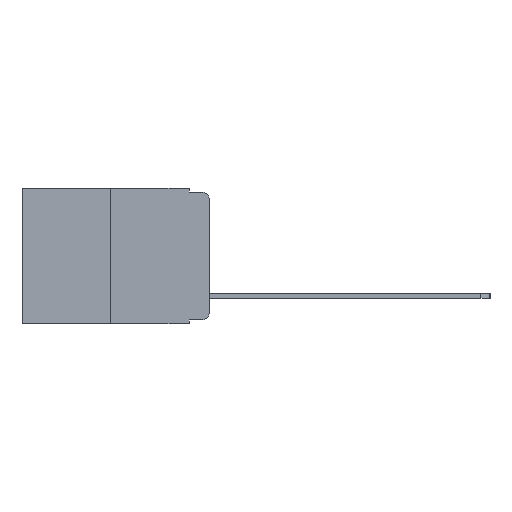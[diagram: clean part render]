
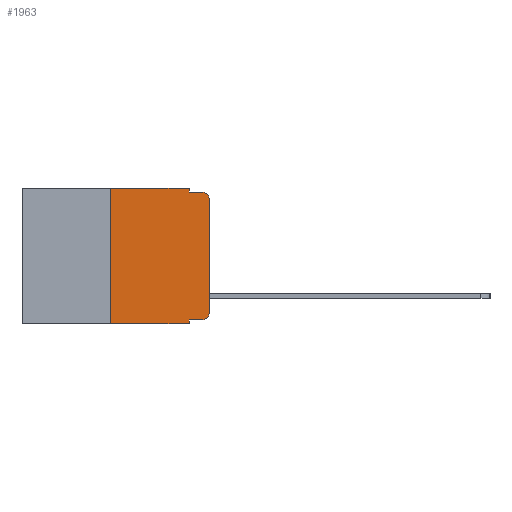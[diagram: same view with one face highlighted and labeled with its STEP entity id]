
A CAD part, left-side view. The second image highlights one B-rep face of the part: STEP entity #1963.
In plain terms, the highlighted planar face has unit normal (-1, 0, 0).
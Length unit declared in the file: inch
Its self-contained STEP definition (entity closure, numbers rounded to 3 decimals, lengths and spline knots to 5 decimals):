
#186 = DIRECTION ( 'NONE',  ( 0., 0., 1. ) ) ;
#354 = CARTESIAN_POINT ( 'NONE',  ( 0., 0.25, 0. ) ) ;
#454 = CARTESIAN_POINT ( 'NONE',  ( 0., 0.051, 0. ) ) ;
#1043 = CARTESIAN_POINT ( 'NONE',  ( 0., 0.02, -0.313 ) ) ;
#1963 = ADVANCED_FACE ( 'NONE', ( #18475 ), #14191, .F. ) ;
#1985 = ORIENTED_EDGE ( 'NONE', *, *, #7393, .T. ) ;
#2136 = DIRECTION ( 'NONE',  ( 1., 0., 0. ) ) ;
#2278 = DIRECTION ( 'NONE',  ( 0., 0., 1. ) ) ;
#2661 = AXIS2_PLACEMENT_3D ( 'NONE', #5911, #2136, #14071 ) ;
#2663 = CARTESIAN_POINT ( 'NONE',  ( 0., 0.02, -0.333 ) ) ;
#2836 = VERTEX_POINT ( 'NONE', #2663 ) ;
#3315 = AXIS2_PLACEMENT_3D ( 'NONE', #15085, #21780, #11551 ) ;
#3350 = EDGE_CURVE ( 'NONE', #8012, #16950, #9375, .T. ) ;
#3798 = EDGE_CURVE ( 'NONE', #2836, #16119, #5721, .T. ) ;
#3980 = EDGE_CURVE ( 'NONE', #20846, #5091, #10677, .T. ) ;
#4271 = DIRECTION ( 'NONE',  ( 0., 0., -1. ) ) ;
#5091 = VERTEX_POINT ( 'NONE', #18103 ) ;
#5386 = ORIENTED_EDGE ( 'NONE', *, *, #3980, .T. ) ;
#5599 = VECTOR ( 'NONE', #2278, 39.37008 ) ;
#5721 = CIRCLE ( 'NONE', #10090, 0.02 ) ;
#5911 = CARTESIAN_POINT ( 'NONE',  ( 0., 0.473, 0. ) ) ;
#6305 = LINE ( 'NONE', #6767, #14699 ) ;
#6406 = CARTESIAN_POINT ( 'NONE',  ( 0., 0.051, -0.01 ) ) ;
#6421 = ORIENTED_EDGE ( 'NONE', *, *, #3350, .T. ) ;
#6767 = CARTESIAN_POINT ( 'NONE',  ( 0., 0.051, -0.333 ) ) ;
#6988 = EDGE_CURVE ( 'NONE', #16119, #8012, #14178, .T. ) ;
#7312 = ORIENTED_EDGE ( 'NONE', *, *, #13431, .F. ) ;
#7393 = EDGE_CURVE ( 'NONE', #10416, #2836, #6305, .T. ) ;
#7529 = CARTESIAN_POINT ( 'NONE',  ( 0., 0., 0. ) ) ;
#7538 = ORIENTED_EDGE ( 'NONE', *, *, #14615, .F. ) ;
#7574 = EDGE_LOOP ( 'NONE', ( #19333, #6421, #14549, #7538, #20152, #7312, #5386, #12990, #1985, #10213 ) ) ;
#8012 = VERTEX_POINT ( 'NONE', #19024 ) ;
#8112 = LINE ( 'NONE', #11455, #21451 ) ;
#8447 = DIRECTION ( 'NONE',  ( 0., -1., 0. ) ) ;
#9168 = LINE ( 'NONE', #14069, #21903 ) ;
#9375 = CIRCLE ( 'NONE', #3315, 0.02 ) ;
#9409 = VECTOR ( 'NONE', #186, 39.37008 ) ;
#9461 = LINE ( 'NONE', #454, #18765 ) ;
#9604 = DIRECTION ( 'NONE',  ( 0., 0., -1. ) ) ;
#9836 = EDGE_CURVE ( 'NONE', #10416, #5091, #8112, .T. ) ;
#10090 = AXIS2_PLACEMENT_3D ( 'NONE', #1043, #11986, #22185 ) ;
#10213 = ORIENTED_EDGE ( 'NONE', *, *, #3798, .T. ) ;
#10416 = VERTEX_POINT ( 'NONE', #19391 ) ;
#10677 = LINE ( 'NONE', #14719, #13725 ) ;
#11455 = CARTESIAN_POINT ( 'NONE',  ( 0., 0.051, 0. ) ) ;
#11551 = DIRECTION ( 'NONE',  ( 0., 0., -1. ) ) ;
#11986 = DIRECTION ( 'NONE',  ( -1., 0., 0. ) ) ;
#12121 = CARTESIAN_POINT ( 'NONE',  ( 0., 0., -0.313 ) ) ;
#12556 = CARTESIAN_POINT ( 'NONE',  ( 0., 0.25, -0.343 ) ) ;
#12990 = ORIENTED_EDGE ( 'NONE', *, *, #9836, .F. ) ;
#13255 = VERTEX_POINT ( 'NONE', #22770 ) ;
#13431 = EDGE_CURVE ( 'NONE', #20846, #14871, #15656, .T. ) ;
#13725 = VECTOR ( 'NONE', #8447, 39.37008 ) ;
#14069 = CARTESIAN_POINT ( 'NONE',  ( 0., 0.051, -0.01 ) ) ;
#14071 = DIRECTION ( 'NONE',  ( 0., 0., -1. ) ) ;
#14178 = LINE ( 'NONE', #7529, #9409 ) ;
#14191 = PLANE ( 'NONE',  #2661 ) ;
#14229 = VECTOR ( 'NONE', #20067, 39.37008 ) ;
#14549 = ORIENTED_EDGE ( 'NONE', *, *, #18069, .F. ) ;
#14615 = EDGE_CURVE ( 'NONE', #13255, #19472, #9461, .T. ) ;
#14699 = VECTOR ( 'NONE', #20732, 39.37008 ) ;
#14719 = CARTESIAN_POINT ( 'NONE',  ( 0., 0.473, -0.343 ) ) ;
#14871 = VERTEX_POINT ( 'NONE', #20670 ) ;
#15085 = CARTESIAN_POINT ( 'NONE',  ( 0., 0.02, -0.03 ) ) ;
#15256 = EDGE_CURVE ( 'NONE', #14871, #13255, #18769, .T. ) ;
#15656 = LINE ( 'NONE', #354, #5599 ) ;
#15823 = DIRECTION ( 'NONE',  ( 0., -1., 0. ) ) ;
#16119 = VERTEX_POINT ( 'NONE', #12121 ) ;
#16950 = VERTEX_POINT ( 'NONE', #22647 ) ;
#18069 = EDGE_CURVE ( 'NONE', #19472, #16950, #9168, .T. ) ;
#18103 = CARTESIAN_POINT ( 'NONE',  ( 0., 0.051, -0.343 ) ) ;
#18403 = CARTESIAN_POINT ( 'NONE',  ( 0., 0.473, 0. ) ) ;
#18475 = FACE_OUTER_BOUND ( 'NONE', #7574, .T. ) ;
#18765 = VECTOR ( 'NONE', #9604, 39.37008 ) ;
#18769 = LINE ( 'NONE', #18403, #14229 ) ;
#19024 = CARTESIAN_POINT ( 'NONE',  ( 0., 0., -0.03 ) ) ;
#19333 = ORIENTED_EDGE ( 'NONE', *, *, #6988, .T. ) ;
#19391 = CARTESIAN_POINT ( 'NONE',  ( 0., 0.051, -0.333 ) ) ;
#19472 = VERTEX_POINT ( 'NONE', #6406 ) ;
#20067 = DIRECTION ( 'NONE',  ( 0., -1., 0. ) ) ;
#20152 = ORIENTED_EDGE ( 'NONE', *, *, #15256, .F. ) ;
#20670 = CARTESIAN_POINT ( 'NONE',  ( 0., 0.25, 0. ) ) ;
#20732 = DIRECTION ( 'NONE',  ( 0., -1., 0. ) ) ;
#20846 = VERTEX_POINT ( 'NONE', #12556 ) ;
#21451 = VECTOR ( 'NONE', #4271, 39.37008 ) ;
#21780 = DIRECTION ( 'NONE',  ( -1., 0., 0. ) ) ;
#21903 = VECTOR ( 'NONE', #15823, 39.37008 ) ;
#22185 = DIRECTION ( 'NONE',  ( 0., 0., -1. ) ) ;
#22647 = CARTESIAN_POINT ( 'NONE',  ( 0., 0.02, -0.01 ) ) ;
#22770 = CARTESIAN_POINT ( 'NONE',  ( 0., 0.051, 0. ) ) ;
